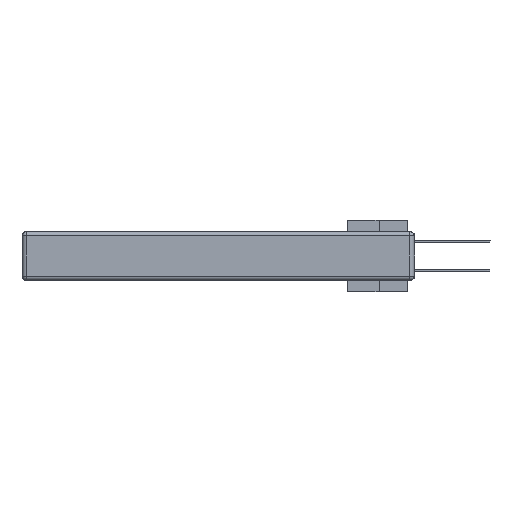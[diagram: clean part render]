
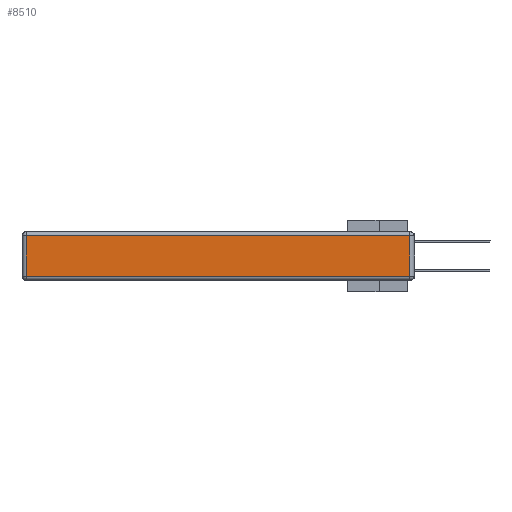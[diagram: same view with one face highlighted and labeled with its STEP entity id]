
A CAD part, left-side view. The second image highlights one B-rep face of the part: STEP entity #8510.
In plain terms, the highlighted planar face has unit normal (-1, 0, 0).
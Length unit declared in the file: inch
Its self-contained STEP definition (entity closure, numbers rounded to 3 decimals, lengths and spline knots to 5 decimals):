
#278 = LINE ( 'NONE', #22697, #11937 ) ;
#821 = ORIENTED_EDGE ( 'NONE', *, *, #3721, .T. ) ;
#2903 = CARTESIAN_POINT ( 'NONE',  ( 0., 0., -0.343 ) ) ;
#3721 = EDGE_CURVE ( 'NONE', #10583, #5759, #15726, .T. ) ;
#3852 = VERTEX_POINT ( 'NONE', #27091 ) ;
#5759 = VERTEX_POINT ( 'NONE', #11821 ) ;
#6898 = EDGE_CURVE ( 'NONE', #3852, #10583, #22638, .T. ) ;
#8510 = ADVANCED_FACE ( 'NONE', ( #16875 ), #13767, .T. ) ;
#8685 = VECTOR ( 'NONE', #12802, 39.37008 ) ;
#10583 = VERTEX_POINT ( 'NONE', #35473 ) ;
#11821 = CARTESIAN_POINT ( 'NONE',  ( 0., 2.72, -0.313 ) ) ;
#11937 = VECTOR ( 'NONE', #33879, 39.37008 ) ;
#12802 = DIRECTION ( 'NONE',  ( 0., 0., -1. ) ) ;
#13767 = PLANE ( 'NONE',  #19850 ) ;
#15066 = EDGE_CURVE ( 'NONE', #31054, #3852, #278, .T. ) ;
#15726 = LINE ( 'NONE', #18653, #8685 ) ;
#16678 = CARTESIAN_POINT ( 'NONE',  ( 0., 0., -0.313 ) ) ;
#16783 = CARTESIAN_POINT ( 'NONE',  ( 0., 2.75, -0.03 ) ) ;
#16875 = FACE_OUTER_BOUND ( 'NONE', #17288, .T. ) ;
#17288 = EDGE_LOOP ( 'NONE', ( #26906, #35070, #23106, #821 ) ) ;
#17498 = DIRECTION ( 'NONE',  ( 0., 1., 0. ) ) ;
#18653 = CARTESIAN_POINT ( 'NONE',  ( 0., 2.72, -0.343 ) ) ;
#19428 = DIRECTION ( 'NONE',  ( 0., 0., 1. ) ) ;
#19850 = AXIS2_PLACEMENT_3D ( 'NONE', #2903, #28048, #19428 ) ;
#19857 = VECTOR ( 'NONE', #30966, 39.37008 ) ;
#22170 = LINE ( 'NONE', #16678, #19857 ) ;
#22638 = LINE ( 'NONE', #16783, #25570 ) ;
#22697 = CARTESIAN_POINT ( 'NONE',  ( 0., 0.03, -0.343 ) ) ;
#23106 = ORIENTED_EDGE ( 'NONE', *, *, #6898, .T. ) ;
#25570 = VECTOR ( 'NONE', #17498, 39.37008 ) ;
#26906 = ORIENTED_EDGE ( 'NONE', *, *, #35718, .T. ) ;
#27091 = CARTESIAN_POINT ( 'NONE',  ( 0., 0.03, -0.03 ) ) ;
#28048 = DIRECTION ( 'NONE',  ( -1., 0., 0. ) ) ;
#29408 = CARTESIAN_POINT ( 'NONE',  ( 0., 0.03, -0.313 ) ) ;
#30966 = DIRECTION ( 'NONE',  ( 0., -1., 0. ) ) ;
#31054 = VERTEX_POINT ( 'NONE', #29408 ) ;
#33879 = DIRECTION ( 'NONE',  ( 0., 0., 1. ) ) ;
#35070 = ORIENTED_EDGE ( 'NONE', *, *, #15066, .T. ) ;
#35473 = CARTESIAN_POINT ( 'NONE',  ( 0., 2.72, -0.03 ) ) ;
#35718 = EDGE_CURVE ( 'NONE', #5759, #31054, #22170, .T. ) ;
